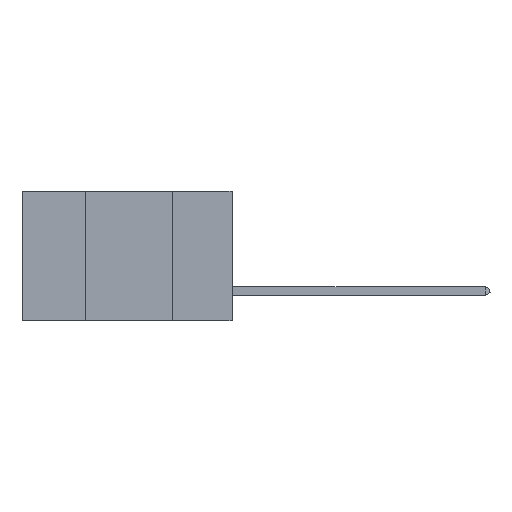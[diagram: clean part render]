
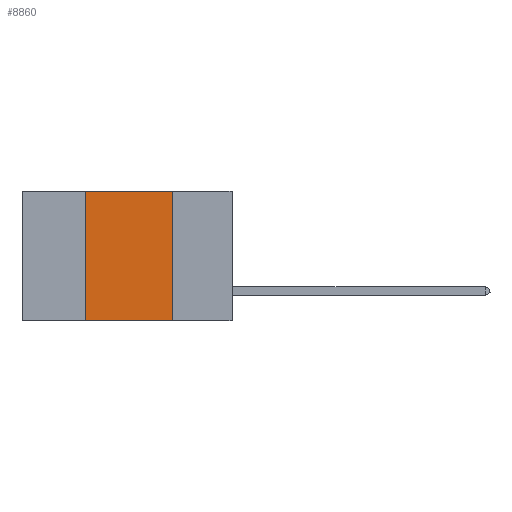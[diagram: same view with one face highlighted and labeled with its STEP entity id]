
A CAD part, left-side view. The second image highlights one B-rep face of the part: STEP entity #8860.
In plain terms, the highlighted planar face has unit normal (-1, 0, 0).
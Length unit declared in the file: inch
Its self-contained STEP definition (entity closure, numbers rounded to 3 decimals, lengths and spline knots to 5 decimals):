
#96 = CARTESIAN_POINT ( 'NONE',  ( 0., 0.6, 0. ) ) ;
#166 = EDGE_CURVE ( 'NONE', #10883, #12856, #7326, .T. ) ;
#1120 = LINE ( 'NONE', #96, #11481 ) ;
#1330 = ORIENTED_EDGE ( 'NONE', *, *, #5435, .F. ) ;
#1673 = CARTESIAN_POINT ( 'NONE',  ( 0., 0.42, -0.37 ) ) ;
#1901 = AXIS2_PLACEMENT_3D ( 'NONE', #12379, #3474, #10489 ) ;
#2898 = FACE_OUTER_BOUND ( 'NONE', #8349, .T. ) ;
#3001 = DIRECTION ( 'NONE',  ( 0., 0., 1. ) ) ;
#3231 = ORIENTED_EDGE ( 'NONE', *, *, #166, .F. ) ;
#3400 = CARTESIAN_POINT ( 'NONE',  ( 0., 0.42, 0. ) ) ;
#3474 = DIRECTION ( 'NONE',  ( 1., 0., 0. ) ) ;
#4464 = CARTESIAN_POINT ( 'NONE',  ( 0., 0.17, 0. ) ) ;
#4537 = ORIENTED_EDGE ( 'NONE', *, *, #7449, .F. ) ;
#4586 = CARTESIAN_POINT ( 'NONE',  ( 0., 0.17, 0. ) ) ;
#5312 = EDGE_CURVE ( 'NONE', #7812, #12856, #10063, .T. ) ;
#5435 = EDGE_CURVE ( 'NONE', #8270, #10883, #1120, .T. ) ;
#5594 = VECTOR ( 'NONE', #3001, 39.37008 ) ;
#6015 = DIRECTION ( 'NONE',  ( 0., -1., 0. ) ) ;
#6685 = DIRECTION ( 'NONE',  ( 0., 0., -1. ) ) ;
#7326 = LINE ( 'NONE', #4586, #10629 ) ;
#7449 = EDGE_CURVE ( 'NONE', #7812, #8270, #10151, .T. ) ;
#7475 = ORIENTED_EDGE ( 'NONE', *, *, #5312, .T. ) ;
#7812 = VERTEX_POINT ( 'NONE', #1673 ) ;
#8270 = VERTEX_POINT ( 'NONE', #3400 ) ;
#8349 = EDGE_LOOP ( 'NONE', ( #3231, #1330, #4537, #7475 ) ) ;
#8537 = CARTESIAN_POINT ( 'NONE',  ( 0., 0.17, -0.37 ) ) ;
#8785 = CARTESIAN_POINT ( 'NONE',  ( 0., 0.6, -0.37 ) ) ;
#8860 = ADVANCED_FACE ( 'NONE', ( #2898 ), #9527, .F. ) ;
#9527 = PLANE ( 'NONE',  #1901 ) ;
#10063 = LINE ( 'NONE', #8785, #10536 ) ;
#10151 = LINE ( 'NONE', #10894, #5594 ) ;
#10489 = DIRECTION ( 'NONE',  ( 0., 0., -1. ) ) ;
#10536 = VECTOR ( 'NONE', #11894, 39.37008 ) ;
#10629 = VECTOR ( 'NONE', #6685, 39.37008 ) ;
#10883 = VERTEX_POINT ( 'NONE', #4464 ) ;
#10894 = CARTESIAN_POINT ( 'NONE',  ( 0., 0.42, 0. ) ) ;
#11481 = VECTOR ( 'NONE', #6015, 39.37008 ) ;
#11894 = DIRECTION ( 'NONE',  ( 0., -1., 0. ) ) ;
#12379 = CARTESIAN_POINT ( 'NONE',  ( 0., 0.6, 0. ) ) ;
#12856 = VERTEX_POINT ( 'NONE', #8537 ) ;
